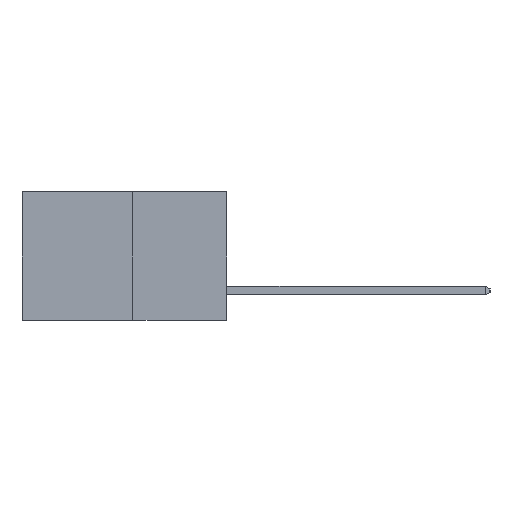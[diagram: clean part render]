
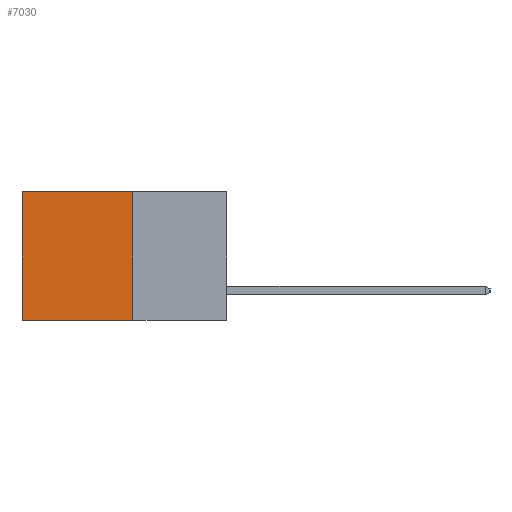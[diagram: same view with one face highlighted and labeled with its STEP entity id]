
A CAD part, left-side view. The second image highlights one B-rep face of the part: STEP entity #7030.
In plain terms, the highlighted planar face has unit normal (-1, 0, 0).
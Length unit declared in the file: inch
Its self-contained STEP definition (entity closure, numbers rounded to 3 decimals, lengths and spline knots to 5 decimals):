
#70 = EDGE_CURVE ( 'NONE', #8397, #853, #19805, .T. ) ;
#627 = PLANE ( 'NONE',  #13385 ) ;
#853 = VERTEX_POINT ( 'NONE', #7124 ) ;
#2423 = LINE ( 'NONE', #16007, #20146 ) ;
#2517 = CARTESIAN_POINT ( 'NONE',  ( 0.277, 0.59, 0. ) ) ;
#3314 = DIRECTION ( 'NONE',  ( 0., 0., -1. ) ) ;
#4111 = DIRECTION ( 'NONE',  ( 1., 0., 0. ) ) ;
#4712 = CARTESIAN_POINT ( 'NONE',  ( 0.277, 0.27, -0.37 ) ) ;
#5271 = ORIENTED_EDGE ( 'NONE', *, *, #7259, .F. ) ;
#5769 = EDGE_LOOP ( 'NONE', ( #22002, #5271, #20863, #16324 ) ) ;
#5829 = CARTESIAN_POINT ( 'NONE',  ( 0.277, 0.59, -0.37 ) ) ;
#6218 = VECTOR ( 'NONE', #18388, 39.37008 ) ;
#6686 = VECTOR ( 'NONE', #18906, 39.37008 ) ;
#6997 = EDGE_CURVE ( 'NONE', #8397, #20414, #2423, .T. ) ;
#7030 = ADVANCED_FACE ( 'NONE', ( #19620 ), #627, .F. ) ;
#7124 = CARTESIAN_POINT ( 'NONE',  ( 0.277, 0.27, -0.37 ) ) ;
#7259 = EDGE_CURVE ( 'NONE', #853, #19715, #19348, .T. ) ;
#8397 = VERTEX_POINT ( 'NONE', #16255 ) ;
#10928 = DIRECTION ( 'NONE',  ( 0., 1., 0. ) ) ;
#12016 = VECTOR ( 'NONE', #3314, 39.37008 ) ;
#13385 = AXIS2_PLACEMENT_3D ( 'NONE', #19491, #4111, #16161 ) ;
#16007 = CARTESIAN_POINT ( 'NONE',  ( 0.277, 0.27, 0. ) ) ;
#16161 = DIRECTION ( 'NONE',  ( 0., 0., -1. ) ) ;
#16255 = CARTESIAN_POINT ( 'NONE',  ( 0.277, 0.27, 0. ) ) ;
#16324 = ORIENTED_EDGE ( 'NONE', *, *, #6997, .T. ) ;
#16963 = CARTESIAN_POINT ( 'NONE',  ( 0.277, 0.59, -0.37 ) ) ;
#18388 = DIRECTION ( 'NONE',  ( 0., 1., 0. ) ) ;
#18906 = DIRECTION ( 'NONE',  ( 0., 0., -1. ) ) ;
#18929 = CARTESIAN_POINT ( 'NONE',  ( 0.277, 0.27, -0.37 ) ) ;
#19348 = LINE ( 'NONE', #4712, #6218 ) ;
#19491 = CARTESIAN_POINT ( 'NONE',  ( 0.277, 0.27, -0.37 ) ) ;
#19620 = FACE_OUTER_BOUND ( 'NONE', #5769, .T. ) ;
#19715 = VERTEX_POINT ( 'NONE', #5829 ) ;
#19805 = LINE ( 'NONE', #18929, #6686 ) ;
#20146 = VECTOR ( 'NONE', #10928, 39.37008 ) ;
#20414 = VERTEX_POINT ( 'NONE', #2517 ) ;
#20863 = ORIENTED_EDGE ( 'NONE', *, *, #70, .F. ) ;
#21081 = LINE ( 'NONE', #16963, #12016 ) ;
#22002 = ORIENTED_EDGE ( 'NONE', *, *, #22098, .T. ) ;
#22098 = EDGE_CURVE ( 'NONE', #20414, #19715, #21081, .T. ) ;
